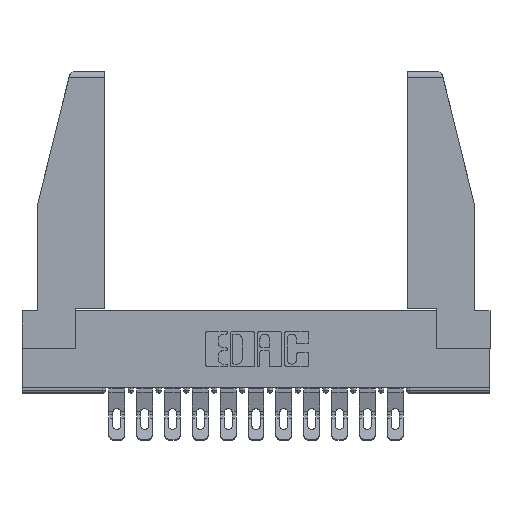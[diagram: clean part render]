
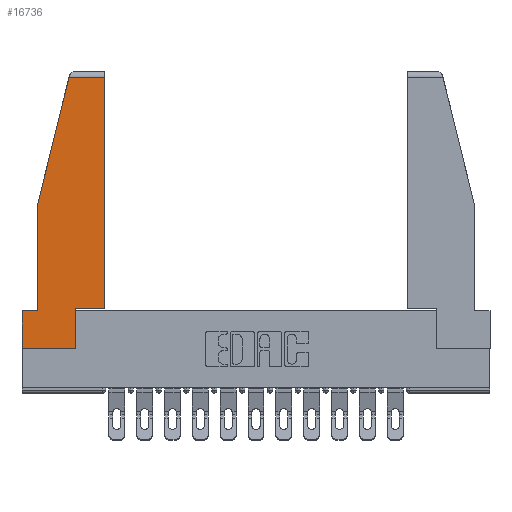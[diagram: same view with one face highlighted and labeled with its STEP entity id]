
A CAD part, top view. The second image highlights one B-rep face of the part: STEP entity #16736.
In plain terms, the highlighted planar face has unit normal (0, 0, 1).
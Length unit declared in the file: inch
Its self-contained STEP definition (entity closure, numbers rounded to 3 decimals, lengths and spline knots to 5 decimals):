
#313 = VECTOR ( 'NONE', #1327, 39.37008 ) ;
#539 = ORIENTED_EDGE ( 'NONE', *, *, #14318, .T. ) ;
#831 = VERTEX_POINT ( 'NONE', #15491 ) ;
#1036 = ORIENTED_EDGE ( 'NONE', *, *, #12244, .T. ) ;
#1068 = AXIS2_PLACEMENT_3D ( 'NONE', #9810, #5510, #12725 ) ;
#1146 = VERTEX_POINT ( 'NONE', #7462 ) ;
#1267 = CARTESIAN_POINT ( 'NONE',  ( 0.271, 1.55, 0. ) ) ;
#1327 = DIRECTION ( 'NONE',  ( 0., -1., 0. ) ) ;
#1561 = CARTESIAN_POINT ( 'NONE',  ( 0.461, 0.223, 0. ) ) ;
#1638 = EDGE_CURVE ( 'NONE', #9289, #12564, #17100, .T. ) ;
#1905 = EDGE_CURVE ( 'NONE', #18235, #2138, #17765, .T. ) ;
#1938 = VERTEX_POINT ( 'NONE', #5334 ) ;
#2048 = CARTESIAN_POINT ( 'NONE',  ( 0.461, 0.223, 0. ) ) ;
#2138 = VERTEX_POINT ( 'NONE', #11712 ) ;
#2374 = VECTOR ( 'NONE', #9969, 39.37008 ) ;
#3233 = DIRECTION ( 'NONE',  ( -1., 0., 0. ) ) ;
#4056 = ORIENTED_EDGE ( 'NONE', *, *, #14962, .T. ) ;
#4716 = CARTESIAN_POINT ( 'NONE',  ( 0.461, 1.52, 0. ) ) ;
#4769 = VECTOR ( 'NONE', #3233, 39.37008 ) ;
#5334 = CARTESIAN_POINT ( 'NONE',  ( 0.086, 0.8, 0. ) ) ;
#5425 = ORIENTED_EDGE ( 'NONE', *, *, #12983, .T. ) ;
#5510 = DIRECTION ( 'NONE',  ( 0., 0., 1. ) ) ;
#5546 = ORIENTED_EDGE ( 'NONE', *, *, #6368, .T. ) ;
#5649 = CARTESIAN_POINT ( 'NONE',  ( 0.297, 0.223, 0. ) ) ;
#5695 = CARTESIAN_POINT ( 'NONE',  ( 0., 0.21, 0. ) ) ;
#6273 = CARTESIAN_POINT ( 'NONE',  ( 0., 0., 0. ) ) ;
#6368 = EDGE_CURVE ( 'NONE', #1938, #18235, #7327, .T. ) ;
#6427 = ORIENTED_EDGE ( 'NONE', *, *, #8462, .T. ) ;
#7060 = VERTEX_POINT ( 'NONE', #6273 ) ;
#7327 = LINE ( 'NONE', #14141, #16879 ) ;
#7462 = CARTESIAN_POINT ( 'NONE',  ( 0.2636, 1.52, 0. ) ) ;
#7615 = LINE ( 'NONE', #15012, #2374 ) ;
#7843 = ORIENTED_EDGE ( 'NONE', *, *, #1638, .T. ) ;
#7858 = DIRECTION ( 'NONE',  ( 0., -1., 0. ) ) ;
#8400 = PLANE ( 'NONE',  #1068 ) ;
#8402 = LINE ( 'NONE', #18006, #9093 ) ;
#8462 = EDGE_CURVE ( 'NONE', #12564, #1146, #13374, .T. ) ;
#9030 = CARTESIAN_POINT ( 'NONE',  ( 0.297, 0., 0. ) ) ;
#9033 = VECTOR ( 'NONE', #17493, 39.37008 ) ;
#9093 = VECTOR ( 'NONE', #10719, 39.37008 ) ;
#9289 = VERTEX_POINT ( 'NONE', #1561 ) ;
#9810 = CARTESIAN_POINT ( 'NONE',  ( 0., 0., 0. ) ) ;
#9969 = DIRECTION ( 'NONE',  ( 1., 0., 0. ) ) ;
#10179 = EDGE_CURVE ( 'NONE', #1146, #1938, #13129, .T. ) ;
#10466 = CARTESIAN_POINT ( 'NONE',  ( 0., 1.52, 0. ) ) ;
#10622 = FACE_OUTER_BOUND ( 'NONE', #12404, .T. ) ;
#10719 = DIRECTION ( 'NONE',  ( 0., 1., 0. ) ) ;
#11712 = CARTESIAN_POINT ( 'NONE',  ( 0., 0.21, 0. ) ) ;
#11738 = ORIENTED_EDGE ( 'NONE', *, *, #10179, .T. ) ;
#11866 = LINE ( 'NONE', #5695, #313 ) ;
#12244 = EDGE_CURVE ( 'NONE', #7060, #13634, #7615, .T. ) ;
#12404 = EDGE_LOOP ( 'NONE', ( #7843, #6427, #11738, #5546, #16718, #5425, #1036, #4056, #539 ) ) ;
#12564 = VERTEX_POINT ( 'NONE', #4716 ) ;
#12725 = DIRECTION ( 'NONE',  ( 1., 0., 0. ) ) ;
#12983 = EDGE_CURVE ( 'NONE', #2138, #7060, #11866, .T. ) ;
#13129 = LINE ( 'NONE', #1267, #9033 ) ;
#13374 = LINE ( 'NONE', #10466, #4769 ) ;
#13634 = VERTEX_POINT ( 'NONE', #9030 ) ;
#13674 = DIRECTION ( 'NONE',  ( 0., 1., 0. ) ) ;
#13901 = VECTOR ( 'NONE', #18246, 39.37008 ) ;
#14081 = CARTESIAN_POINT ( 'NONE',  ( 0., 0.21, 0. ) ) ;
#14141 = CARTESIAN_POINT ( 'NONE',  ( 0.086, 0.8, 0. ) ) ;
#14318 = EDGE_CURVE ( 'NONE', #831, #9289, #18178, .T. ) ;
#14962 = EDGE_CURVE ( 'NONE', #13634, #831, #8402, .T. ) ;
#15012 = CARTESIAN_POINT ( 'NONE',  ( 0., 0., 0. ) ) ;
#15491 = CARTESIAN_POINT ( 'NONE',  ( 0.297, 0.223, 0. ) ) ;
#15541 = DIRECTION ( 'NONE',  ( 1., 0., 0. ) ) ;
#16718 = ORIENTED_EDGE ( 'NONE', *, *, #1905, .T. ) ;
#16736 = ADVANCED_FACE ( 'NONE', ( #10622 ), #8400, .T. ) ;
#16879 = VECTOR ( 'NONE', #7858, 39.37008 ) ;
#17100 = LINE ( 'NONE', #2048, #17991 ) ;
#17493 = DIRECTION ( 'NONE',  ( -0.239, -0.971, 0. ) ) ;
#17523 = VECTOR ( 'NONE', #15541, 39.37008 ) ;
#17765 = LINE ( 'NONE', #14081, #13901 ) ;
#17991 = VECTOR ( 'NONE', #13674, 39.37008 ) ;
#18006 = CARTESIAN_POINT ( 'NONE',  ( 0.297, 0., 0. ) ) ;
#18178 = LINE ( 'NONE', #5649, #17523 ) ;
#18235 = VERTEX_POINT ( 'NONE', #18774 ) ;
#18246 = DIRECTION ( 'NONE',  ( -1., 0., 0. ) ) ;
#18774 = CARTESIAN_POINT ( 'NONE',  ( 0.086, 0.21, 0. ) ) ;
